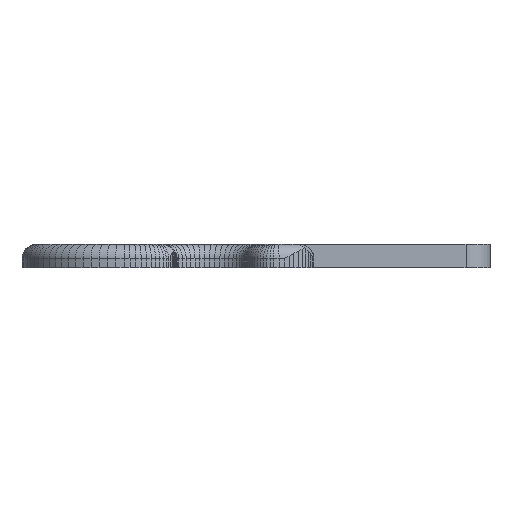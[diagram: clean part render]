
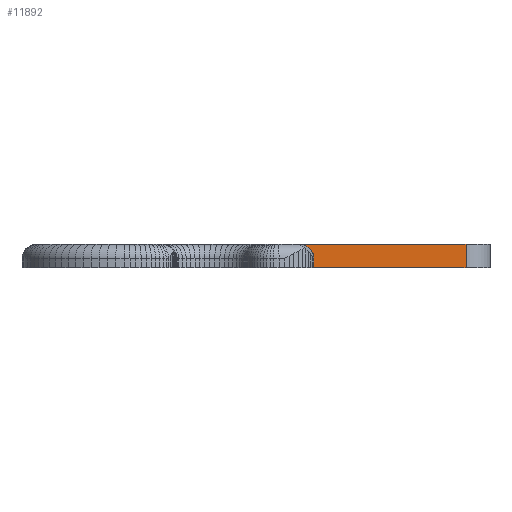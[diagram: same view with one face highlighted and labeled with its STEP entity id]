
A CAD part, front view. The second image highlights one B-rep face of the part: STEP entity #11892.
In plain terms, the highlighted planar face has unit normal (0, -1, 0).
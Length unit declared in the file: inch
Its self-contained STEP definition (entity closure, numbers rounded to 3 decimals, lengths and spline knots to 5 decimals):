
#269 = DIRECTION ( 'NONE',  ( 0., 0., -1. ) ) ;
#787 = EDGE_CURVE ( 'NONE', #1535, #9935, #4403, .T. ) ;
#881 = EDGE_CURVE ( 'NONE', #9935, #6331, #9978, .T. ) ;
#899 = DIRECTION ( 'NONE',  ( 0., -1., 0. ) ) ;
#1245 = VERTEX_POINT ( 'NONE', #4463 ) ;
#1535 = VERTEX_POINT ( 'NONE', #4072 ) ;
#2083 = EDGE_CURVE ( 'NONE', #1535, #1245, #9010, .T. ) ;
#2161 = ORIENTED_EDGE ( 'NONE', *, *, #7270, .T. ) ;
#2436 = DIRECTION ( 'NONE',  ( 0., 0., -1. ) ) ;
#2581 = DIRECTION ( 'NONE',  ( 0., 0., -1. ) ) ;
#3114 = CARTESIAN_POINT ( 'NONE',  ( 0., -0.70627, 0.19685 ) ) ;
#3573 = CARTESIAN_POINT ( 'NONE',  ( -0.17664, -0.70627, 0.0748 ) ) ;
#4072 = CARTESIAN_POINT ( 'NONE',  ( 1.24462, -0.70627, 0.19685 ) ) ;
#4403 = LINE ( 'NONE', #11235, #10342 ) ;
#4463 = CARTESIAN_POINT ( 'NONE',  ( 1.24462, -0.70627, 0. ) ) ;
#4510 = DIRECTION ( 'NONE',  ( 0., 1., 0. ) ) ;
#5000 = CARTESIAN_POINT ( 'NONE',  ( -0.05459, -0.70627, 0. ) ) ;
#5712 = EDGE_LOOP ( 'NONE', ( #14499, #12437, #2161, #13374, #10685 ) ) ;
#5993 = CARTESIAN_POINT ( 'NONE',  ( -0.05459, -0.70627, 0. ) ) ;
#6153 = VERTEX_POINT ( 'NONE', #5000 ) ;
#6331 = VERTEX_POINT ( 'NONE', #8517 ) ;
#6887 = AXIS2_PLACEMENT_3D ( 'NONE', #3114, #899, #7767 ) ;
#7270 = EDGE_CURVE ( 'NONE', #6331, #6153, #11275, .T. ) ;
#7767 = DIRECTION ( 'NONE',  ( 0., 0., -1. ) ) ;
#8517 = CARTESIAN_POINT ( 'NONE',  ( -0.05459, -0.70627, 0.0748 ) ) ;
#8825 = PLANE ( 'NONE',  #6887 ) ;
#9010 = LINE ( 'NONE', #13985, #11786 ) ;
#9069 = AXIS2_PLACEMENT_3D ( 'NONE', #3573, #4510, #2436 ) ;
#9664 = DIRECTION ( 'NONE',  ( -1., 0., 0. ) ) ;
#9935 = VERTEX_POINT ( 'NONE', #14295 ) ;
#9978 = CIRCLE ( 'NONE', #9069, 0.12205 ) ;
#10342 = VECTOR ( 'NONE', #13644, 39.37008 ) ;
#10685 = ORIENTED_EDGE ( 'NONE', *, *, #2083, .F. ) ;
#11235 = CARTESIAN_POINT ( 'NONE',  ( 0., -0.70627, 0.19685 ) ) ;
#11275 = LINE ( 'NONE', #5993, #13289 ) ;
#11786 = VECTOR ( 'NONE', #2581, 39.37008 ) ;
#11892 = ADVANCED_FACE ( 'NONE', ( #12858 ), #8825, .T. ) ;
#12437 = ORIENTED_EDGE ( 'NONE', *, *, #881, .T. ) ;
#12858 = FACE_OUTER_BOUND ( 'NONE', #5712, .T. ) ;
#13289 = VECTOR ( 'NONE', #269, 39.37008 ) ;
#13374 = ORIENTED_EDGE ( 'NONE', *, *, #14165, .F. ) ;
#13644 = DIRECTION ( 'NONE',  ( -1., 0., 0. ) ) ;
#13985 = CARTESIAN_POINT ( 'NONE',  ( 1.24462, -0.70627, 0.19685 ) ) ;
#14165 = EDGE_CURVE ( 'NONE', #1245, #6153, #14894, .T. ) ;
#14191 = VECTOR ( 'NONE', #9664, 39.37008 ) ;
#14225 = CARTESIAN_POINT ( 'NONE',  ( 0., -0.70627, 0. ) ) ;
#14295 = CARTESIAN_POINT ( 'NONE',  ( -0.17664, -0.70627, 0.19685 ) ) ;
#14499 = ORIENTED_EDGE ( 'NONE', *, *, #787, .T. ) ;
#14894 = LINE ( 'NONE', #14225, #14191 ) ;
